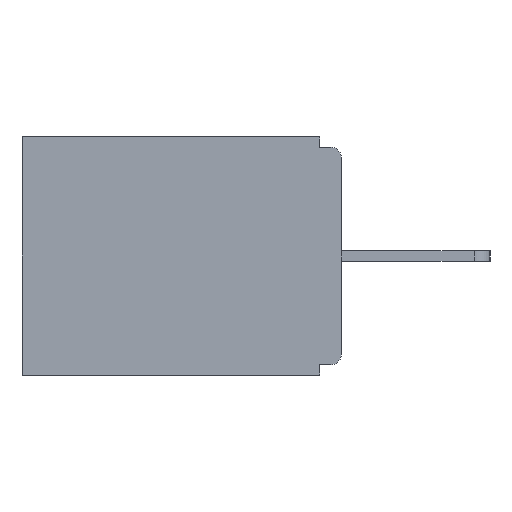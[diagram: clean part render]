
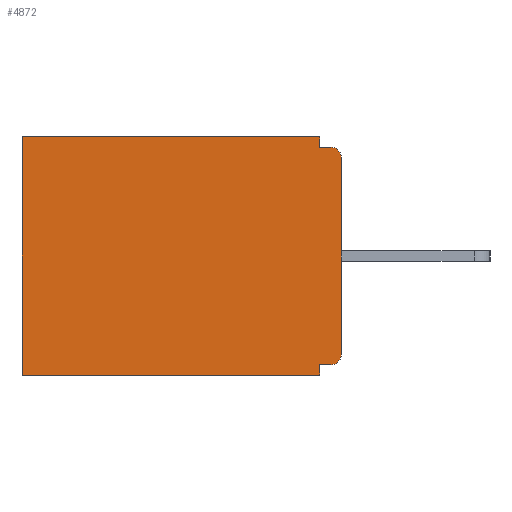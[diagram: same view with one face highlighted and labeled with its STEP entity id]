
A CAD part, left-side view. The second image highlights one B-rep face of the part: STEP entity #4872.
In plain terms, the highlighted planar face has unit normal (-1, 0, 0).
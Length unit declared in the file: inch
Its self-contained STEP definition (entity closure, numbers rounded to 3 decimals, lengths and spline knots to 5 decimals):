
#129 = ORIENTED_EDGE ( 'NONE', *, *, #7877, .T. ) ;
#696 = CARTESIAN_POINT ( 'NONE',  ( 0.298, 0.031, -0.015 ) ) ;
#784 = ORIENTED_EDGE ( 'NONE', *, *, #2687, .T. ) ;
#854 = LINE ( 'NONE', #9686, #9164 ) ;
#895 = LINE ( 'NONE', #2163, #2394 ) ;
#1141 = EDGE_CURVE ( 'NONE', #11184, #10317, #3556, .T. ) ;
#1808 = CARTESIAN_POINT ( 'NONE',  ( 0.298, 0.031, -0.343 ) ) ;
#2008 = DIRECTION ( 'NONE',  ( 0., 0., -1. ) ) ;
#2163 = CARTESIAN_POINT ( 'NONE',  ( 0.298, 0.46, 0. ) ) ;
#2168 = VERTEX_POINT ( 'NONE', #13446 ) ;
#2221 = CARTESIAN_POINT ( 'NONE',  ( 0.298, 0.031, -0.343 ) ) ;
#2250 = LINE ( 'NONE', #9970, #4260 ) ;
#2394 = VECTOR ( 'NONE', #12205, 39.37008 ) ;
#2417 = VECTOR ( 'NONE', #6806, 39.37008 ) ;
#2687 = EDGE_CURVE ( 'NONE', #9128, #11443, #854, .T. ) ;
#2744 = CARTESIAN_POINT ( 'NONE',  ( 0.298, 0.031, -0.328 ) ) ;
#2751 = EDGE_CURVE ( 'NONE', #4747, #2168, #4456, .T. ) ;
#3233 = CARTESIAN_POINT ( 'NONE',  ( 0.298, 0., 0. ) ) ;
#3336 = CARTESIAN_POINT ( 'NONE',  ( 0.298, 0., -0.343 ) ) ;
#3556 = LINE ( 'NONE', #8129, #13325 ) ;
#3645 = AXIS2_PLACEMENT_3D ( 'NONE', #3233, #9109, #3705 ) ;
#3705 = DIRECTION ( 'NONE',  ( 0., 0., -1. ) ) ;
#4051 = EDGE_CURVE ( 'NONE', #10562, #7555, #9260, .T. ) ;
#4260 = VECTOR ( 'NONE', #13646, 39.37008 ) ;
#4456 = LINE ( 'NONE', #3336, #13170 ) ;
#4504 = AXIS2_PLACEMENT_3D ( 'NONE', #5718, #11150, #2008 ) ;
#4747 = VERTEX_POINT ( 'NONE', #1808 ) ;
#4872 = ADVANCED_FACE ( 'NONE', ( #10068 ), #14616, .F. ) ;
#4893 = CARTESIAN_POINT ( 'NONE',  ( 0.298, 0.031, 0. ) ) ;
#4894 = CARTESIAN_POINT ( 'NONE',  ( 0.298, 0.015, -0.313 ) ) ;
#5373 = LINE ( 'NONE', #8601, #8318 ) ;
#5604 = EDGE_CURVE ( 'NONE', #11443, #2168, #895, .T. ) ;
#5718 = CARTESIAN_POINT ( 'NONE',  ( 0.298, 0.015, -0.03 ) ) ;
#5756 = ORIENTED_EDGE ( 'NONE', *, *, #11288, .F. ) ;
#5867 = ORIENTED_EDGE ( 'NONE', *, *, #8173, .T. ) ;
#5917 = ORIENTED_EDGE ( 'NONE', *, *, #2751, .F. ) ;
#5974 = DIRECTION ( 'NONE',  ( 0., 0., -1. ) ) ;
#6415 = AXIS2_PLACEMENT_3D ( 'NONE', #4894, #9524, #12811 ) ;
#6500 = DIRECTION ( 'NONE',  ( 0., 1., 0. ) ) ;
#6586 = EDGE_CURVE ( 'NONE', #9128, #10562, #2250, .T. ) ;
#6806 = DIRECTION ( 'NONE',  ( 0., 0., -1. ) ) ;
#6870 = CARTESIAN_POINT ( 'NONE',  ( 0.298, 0.015, -0.015 ) ) ;
#6890 = ORIENTED_EDGE ( 'NONE', *, *, #4051, .F. ) ;
#7466 = DIRECTION ( 'NONE',  ( 0., 1., 0. ) ) ;
#7555 = VERTEX_POINT ( 'NONE', #6870 ) ;
#7877 = EDGE_CURVE ( 'NONE', #11618, #10317, #10469, .T. ) ;
#7928 = LINE ( 'NONE', #2221, #2417 ) ;
#8129 = CARTESIAN_POINT ( 'NONE',  ( 0.298, 0., 0. ) ) ;
#8173 = EDGE_CURVE ( 'NONE', #11184, #7555, #10936, .T. ) ;
#8318 = VECTOR ( 'NONE', #7466, 39.37008 ) ;
#8601 = CARTESIAN_POINT ( 'NONE',  ( 0.298, 0., -0.328 ) ) ;
#9026 = DIRECTION ( 'NONE',  ( 0., 1., 0. ) ) ;
#9109 = DIRECTION ( 'NONE',  ( 1., 0., 0. ) ) ;
#9128 = VERTEX_POINT ( 'NONE', #4893 ) ;
#9164 = VECTOR ( 'NONE', #6500, 39.37008 ) ;
#9260 = LINE ( 'NONE', #11779, #10238 ) ;
#9299 = EDGE_LOOP ( 'NONE', ( #5867, #6890, #9559, #784, #11593, #5917, #12325, #5756, #129, #10675 ) ) ;
#9524 = DIRECTION ( 'NONE',  ( -1., 0., 0. ) ) ;
#9559 = ORIENTED_EDGE ( 'NONE', *, *, #6586, .F. ) ;
#9686 = CARTESIAN_POINT ( 'NONE',  ( 0.298, 0., 0. ) ) ;
#9970 = CARTESIAN_POINT ( 'NONE',  ( 0.298, 0.031, -0.343 ) ) ;
#10068 = FACE_OUTER_BOUND ( 'NONE', #9299, .T. ) ;
#10238 = VECTOR ( 'NONE', #14169, 39.37008 ) ;
#10317 = VERTEX_POINT ( 'NONE', #13193 ) ;
#10469 = CIRCLE ( 'NONE', #6415, 0.015 ) ;
#10562 = VERTEX_POINT ( 'NONE', #696 ) ;
#10675 = ORIENTED_EDGE ( 'NONE', *, *, #1141, .F. ) ;
#10936 = CIRCLE ( 'NONE', #4504, 0.015 ) ;
#11026 = EDGE_CURVE ( 'NONE', #12777, #4747, #7928, .T. ) ;
#11150 = DIRECTION ( 'NONE',  ( -1., 0., 0. ) ) ;
#11184 = VERTEX_POINT ( 'NONE', #11736 ) ;
#11288 = EDGE_CURVE ( 'NONE', #11618, #12777, #5373, .T. ) ;
#11443 = VERTEX_POINT ( 'NONE', #13737 ) ;
#11593 = ORIENTED_EDGE ( 'NONE', *, *, #5604, .T. ) ;
#11618 = VERTEX_POINT ( 'NONE', #14112 ) ;
#11736 = CARTESIAN_POINT ( 'NONE',  ( 0.298, 0., -0.03 ) ) ;
#11779 = CARTESIAN_POINT ( 'NONE',  ( 0.298, 0., -0.015 ) ) ;
#12205 = DIRECTION ( 'NONE',  ( 0., 0., -1. ) ) ;
#12325 = ORIENTED_EDGE ( 'NONE', *, *, #11026, .F. ) ;
#12777 = VERTEX_POINT ( 'NONE', #2744 ) ;
#12811 = DIRECTION ( 'NONE',  ( 0., 0., -1. ) ) ;
#13170 = VECTOR ( 'NONE', #9026, 39.37008 ) ;
#13193 = CARTESIAN_POINT ( 'NONE',  ( 0.298, 0., -0.313 ) ) ;
#13325 = VECTOR ( 'NONE', #5974, 39.37008 ) ;
#13446 = CARTESIAN_POINT ( 'NONE',  ( 0.298, 0.46, -0.343 ) ) ;
#13646 = DIRECTION ( 'NONE',  ( 0., 0., -1. ) ) ;
#13737 = CARTESIAN_POINT ( 'NONE',  ( 0.298, 0.46, 0. ) ) ;
#14112 = CARTESIAN_POINT ( 'NONE',  ( 0.298, 0.015, -0.328 ) ) ;
#14169 = DIRECTION ( 'NONE',  ( 0., -1., 0. ) ) ;
#14616 = PLANE ( 'NONE',  #3645 ) ;
